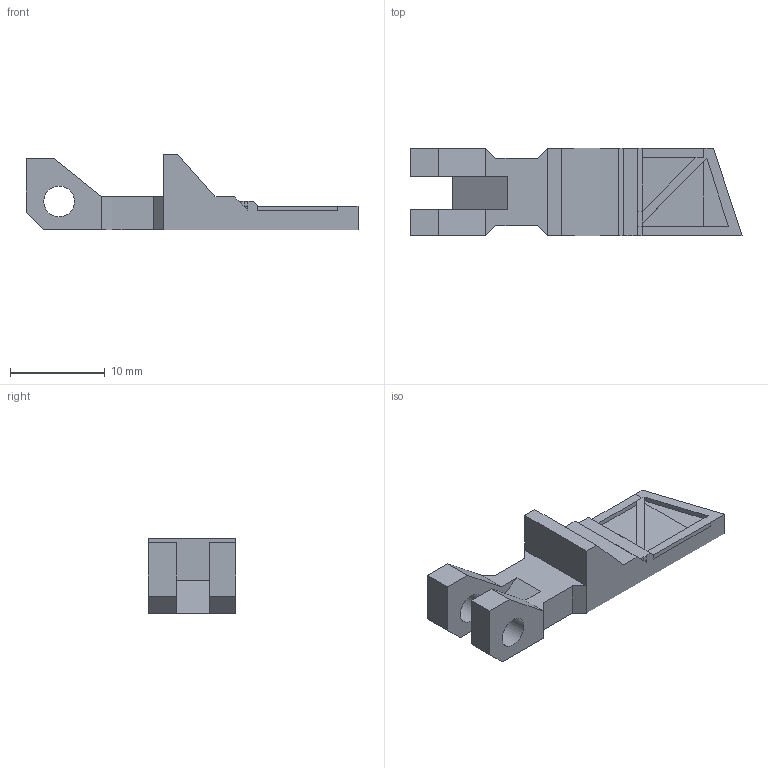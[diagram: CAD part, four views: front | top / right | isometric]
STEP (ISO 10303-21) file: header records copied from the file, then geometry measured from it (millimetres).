
FILE_DESCRIPTION(/* description */ (''),/* implementation_level */ '2;1');
FILE_NAME(/* name */ 'latte bar.step',/* time_stamp */ '2021-05-31T19:21:55-06:00',/* author */ (''),/* organization */ (''),/* preprocessor_version */ 'ST-DEVELOPER v18.1',/* originating_system */ 'Autodesk Translation Framework v10.9.0.1377',/* authorisation */ '');
FILE_SCHEMA (('AUTOMOTIVE_DESIGN { 1 0 10303 214 3 1 1 }'));
Length unit declared in the file: millimetre
Products named in the file (1): low pro bar mag release
Bounding box: 35.03 x 9.25 x 8 mm (x, y, z)
Volume: 1047.2 mm3; surface area: 1135.4 mm2
Topology: 1 solids, 1 shells, 55 faces, 149 edges, 96 vertices
Faces by surface type: plane 53, cylinder 2
Full cylindrical faces by diameter (mm): 3.25 x2
Entity records: 1728 total; most frequent: CARTESIAN_POINT 301, ORIENTED_EDGE 298, DIRECTION 265, EDGE_CURVE 149, LINE 145, VECTOR 145, VERTEX_POINT 96, AXIS2_PLACEMENT_3D 60
